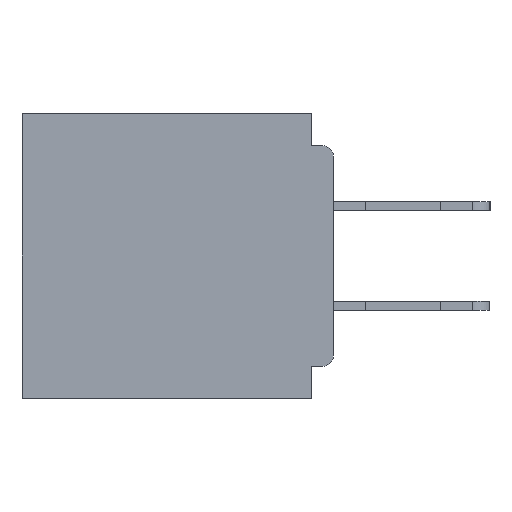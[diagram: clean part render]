
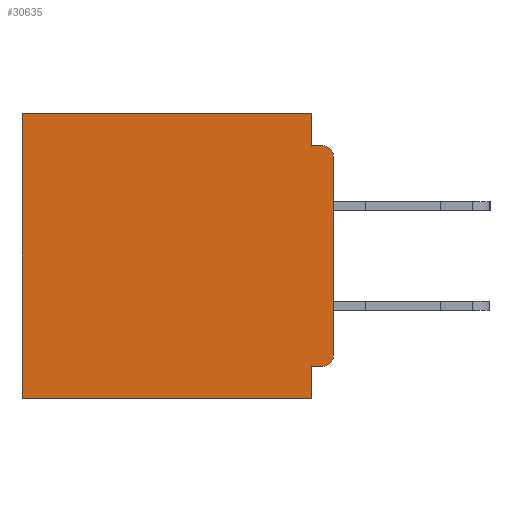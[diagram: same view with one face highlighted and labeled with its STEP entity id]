
A CAD part, left-side view. The second image highlights one B-rep face of the part: STEP entity #30635.
In plain terms, the highlighted planar face has unit normal (-1, 0, 0).
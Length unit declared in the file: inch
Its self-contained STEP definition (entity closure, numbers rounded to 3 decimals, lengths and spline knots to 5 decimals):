
#334 = DIRECTION ( 'NONE',  ( 0., 1., 0. ) ) ;
#1893 = ORIENTED_EDGE ( 'NONE', *, *, #4434, .F. ) ;
#3770 = ORIENTED_EDGE ( 'NONE', *, *, #28046, .T. ) ;
#3847 = VECTOR ( 'NONE', #43312, 39.37008 ) ;
#3892 = VERTEX_POINT ( 'NONE', #43921 ) ;
#4289 = VERTEX_POINT ( 'NONE', #20511 ) ;
#4434 = EDGE_CURVE ( 'NONE', #33624, #19135, #13031, .T. ) ;
#4821 = CARTESIAN_POINT ( 'NONE',  ( 0.3, 0.031, 0. ) ) ;
#5587 = DIRECTION ( 'NONE',  ( 0., 0., -1. ) ) ;
#5872 = CARTESIAN_POINT ( 'NONE',  ( 0.3, 0.015, -0.34 ) ) ;
#6077 = LINE ( 'NONE', #42974, #50584 ) ;
#6379 = ORIENTED_EDGE ( 'NONE', *, *, #45477, .F. ) ;
#7355 = ORIENTED_EDGE ( 'NONE', *, *, #37872, .F. ) ;
#8876 = ORIENTED_EDGE ( 'NONE', *, *, #42487, .F. ) ;
#9289 = DIRECTION ( 'NONE',  ( 0., 0., -1. ) ) ;
#10038 = DIRECTION ( 'NONE',  ( 0., 0., -1. ) ) ;
#11733 = VECTOR ( 'NONE', #5587, 39.37008 ) ;
#11843 = LINE ( 'NONE', #20059, #21574 ) ;
#13031 = LINE ( 'NONE', #4821, #11733 ) ;
#14303 = ORIENTED_EDGE ( 'NONE', *, *, #30289, .T. ) ;
#14512 = DIRECTION ( 'NONE',  ( -1., 0., 0. ) ) ;
#14837 = LINE ( 'NONE', #39244, #3847 ) ;
#15898 = DIRECTION ( 'NONE',  ( 0., -1., 0. ) ) ;
#19135 = VERTEX_POINT ( 'NONE', #49897 ) ;
#20059 = CARTESIAN_POINT ( 'NONE',  ( 0.3, 0., -0.045 ) ) ;
#20511 = CARTESIAN_POINT ( 'NONE',  ( 0.3, 0.437, -0.4 ) ) ;
#20939 = CARTESIAN_POINT ( 'NONE',  ( 0.3, 0., -0.355 ) ) ;
#21574 = VECTOR ( 'NONE', #15898, 39.37008 ) ;
#23791 = AXIS2_PLACEMENT_3D ( 'NONE', #40789, #48822, #24733 ) ;
#24174 = CARTESIAN_POINT ( 'NONE',  ( 0.3, 0.031, -0.355 ) ) ;
#24461 = VERTEX_POINT ( 'NONE', #49074 ) ;
#24577 = EDGE_CURVE ( 'NONE', #41200, #25276, #47494, .T. ) ;
#24733 = DIRECTION ( 'NONE',  ( 0., 0., -1. ) ) ;
#25276 = VERTEX_POINT ( 'NONE', #30161 ) ;
#26571 = ORIENTED_EDGE ( 'NONE', *, *, #42420, .T. ) ;
#26930 = DIRECTION ( 'NONE',  ( 0., 0., -1. ) ) ;
#27510 = AXIS2_PLACEMENT_3D ( 'NONE', #38879, #14512, #42943 ) ;
#27851 = EDGE_CURVE ( 'NONE', #37214, #24461, #31709, .T. ) ;
#27857 = VERTEX_POINT ( 'NONE', #46666 ) ;
#28046 = EDGE_CURVE ( 'NONE', #33624, #3892, #43062, .T. ) ;
#28970 = LINE ( 'NONE', #35681, #42170 ) ;
#30161 = CARTESIAN_POINT ( 'NONE',  ( 0.3, 0.031, -0.4 ) ) ;
#30289 = EDGE_CURVE ( 'NONE', #40859, #27857, #36453, .T. ) ;
#30608 = VECTOR ( 'NONE', #334, 39.37008 ) ;
#30635 = ADVANCED_FACE ( 'NONE', ( #33281 ), #44851, .F. ) ;
#31709 = CIRCLE ( 'NONE', #38511, 0.015 ) ;
#31863 = LINE ( 'NONE', #20939, #30608 ) ;
#32646 = ORIENTED_EDGE ( 'NONE', *, *, #49729, .F. ) ;
#33281 = FACE_OUTER_BOUND ( 'NONE', #46626, .T. ) ;
#33624 = VERTEX_POINT ( 'NONE', #50627 ) ;
#33775 = CARTESIAN_POINT ( 'NONE',  ( 0.3, 0.031, -0.4 ) ) ;
#34495 = DIRECTION ( 'NONE',  ( -1., 0., 0. ) ) ;
#35681 = CARTESIAN_POINT ( 'NONE',  ( 0.3, 0., -0.4 ) ) ;
#36453 = CIRCLE ( 'NONE', #27510, 0.015 ) ;
#36795 = VECTOR ( 'NONE', #9289, 39.37008 ) ;
#37214 = VERTEX_POINT ( 'NONE', #48305 ) ;
#37872 = EDGE_CURVE ( 'NONE', #37214, #41200, #31863, .T. ) ;
#38511 = AXIS2_PLACEMENT_3D ( 'NONE', #5872, #34495, #10038 ) ;
#38879 = CARTESIAN_POINT ( 'NONE',  ( 0.3, 0.015, -0.06 ) ) ;
#39244 = CARTESIAN_POINT ( 'NONE',  ( 0.3, 0.437, -0.4 ) ) ;
#39755 = DIRECTION ( 'NONE',  ( 0., 1., 0. ) ) ;
#39795 = CARTESIAN_POINT ( 'NONE',  ( 0.3, 0., 0. ) ) ;
#40789 = CARTESIAN_POINT ( 'NONE',  ( 0.3, 0., -0.4 ) ) ;
#40859 = VERTEX_POINT ( 'NONE', #41494 ) ;
#41200 = VERTEX_POINT ( 'NONE', #24174 ) ;
#41494 = CARTESIAN_POINT ( 'NONE',  ( 0.3, 0., -0.06 ) ) ;
#42170 = VECTOR ( 'NONE', #39755, 39.37008 ) ;
#42420 = EDGE_CURVE ( 'NONE', #3892, #4289, #14837, .T. ) ;
#42487 = EDGE_CURVE ( 'NONE', #25276, #4289, #28970, .T. ) ;
#42943 = DIRECTION ( 'NONE',  ( 0., 0., -1. ) ) ;
#42974 = CARTESIAN_POINT ( 'NONE',  ( 0.3, 0., -0.4 ) ) ;
#43062 = LINE ( 'NONE', #39795, #51134 ) ;
#43312 = DIRECTION ( 'NONE',  ( 0., 0., -1. ) ) ;
#43857 = DIRECTION ( 'NONE',  ( 0., 1., 0. ) ) ;
#43921 = CARTESIAN_POINT ( 'NONE',  ( 0.3, 0.437, 0. ) ) ;
#44553 = ORIENTED_EDGE ( 'NONE', *, *, #27851, .T. ) ;
#44851 = PLANE ( 'NONE',  #23791 ) ;
#45477 = EDGE_CURVE ( 'NONE', #19135, #27857, #11843, .T. ) ;
#46626 = EDGE_LOOP ( 'NONE', ( #32646, #14303, #6379, #1893, #3770, #26571, #8876, #50640, #7355, #44553 ) ) ;
#46666 = CARTESIAN_POINT ( 'NONE',  ( 0.3, 0.015, -0.045 ) ) ;
#47494 = LINE ( 'NONE', #33775, #36795 ) ;
#48305 = CARTESIAN_POINT ( 'NONE',  ( 0.3, 0.015, -0.355 ) ) ;
#48822 = DIRECTION ( 'NONE',  ( 1., 0., 0. ) ) ;
#49074 = CARTESIAN_POINT ( 'NONE',  ( 0.3, 0., -0.34 ) ) ;
#49729 = EDGE_CURVE ( 'NONE', #40859, #24461, #6077, .T. ) ;
#49897 = CARTESIAN_POINT ( 'NONE',  ( 0.3, 0.031, -0.045 ) ) ;
#50584 = VECTOR ( 'NONE', #26930, 39.37008 ) ;
#50627 = CARTESIAN_POINT ( 'NONE',  ( 0.3, 0.031, 0. ) ) ;
#50640 = ORIENTED_EDGE ( 'NONE', *, *, #24577, .F. ) ;
#51134 = VECTOR ( 'NONE', #43857, 39.37008 ) ;
